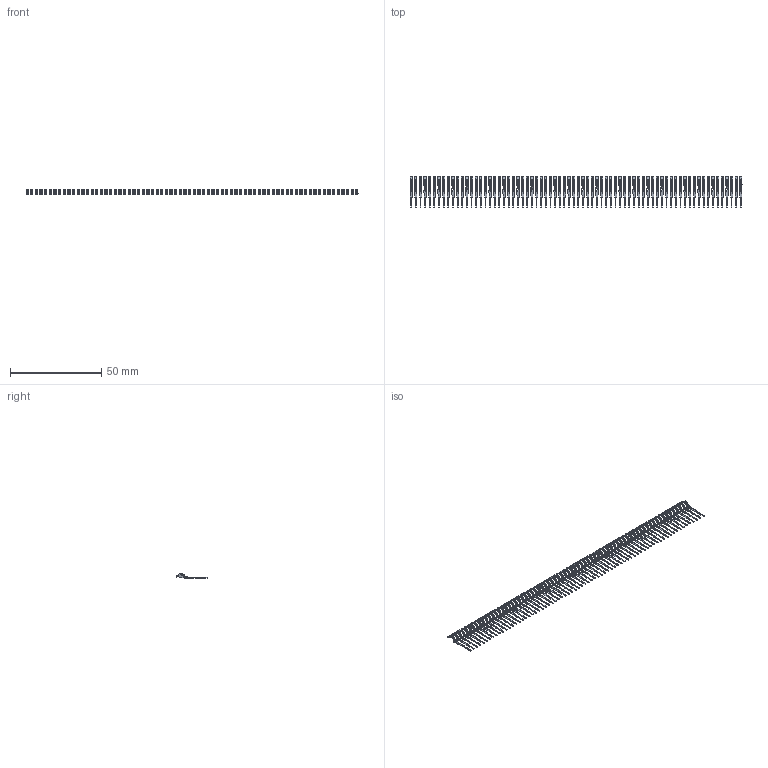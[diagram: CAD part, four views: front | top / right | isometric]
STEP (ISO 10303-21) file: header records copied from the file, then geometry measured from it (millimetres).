
FILE_DESCRIPTION (( 'STEP AP203' ), '1' );
FILE_NAME ('395-072-525-412.STEP', '2020-09-25T07:37:14', ( '' ), ( '' ), 'SwSTEP 2.0', 'SolidWorks 2020', '' );
FILE_SCHEMA (( 'CONFIG_CONTROL_DESIGN' ));
Length unit declared in the file: inch
Products named in the file (3): 395-072-525-412; 345 Part_0.110 Offset - Side Mount; 345-292-001_345-293-125
Assembly tree (73 placements, depth 2):
  395-072-525-412
    345 Part_0.110 Offset - Side Mount
    345-292-001_345-293-125  x72
Bounding box: 181.61 x 17.14 x 2.7 mm (x, y, z)
Surface area: 4181.5 mm2 (no closed solid volume)
Topology: 0 solids, 72 shells, 3312 faces, 8712 edges, 4392 vertices
Faces by surface type: plane 2304, cylinder 1008
Entity records: 50203 total; most frequent: CARTESIAN_POINT 8728, ORIENTED_EDGE 8657, DIRECTION 7579, EDGE_CURVE 4367, LINE 3951, VECTOR 3951, VERTEX_POINT 2906, AXIS2_PLACEMENT_3D 1814
